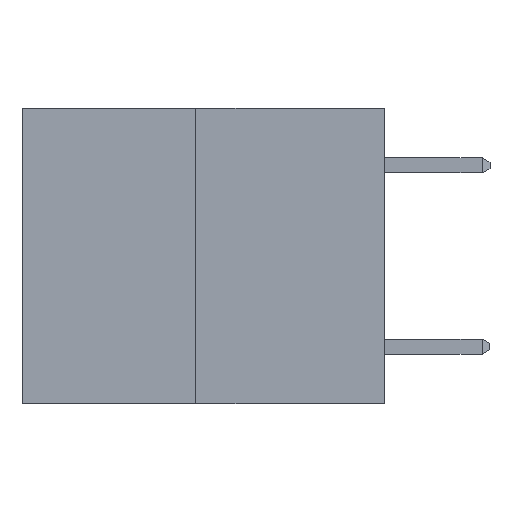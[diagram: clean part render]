
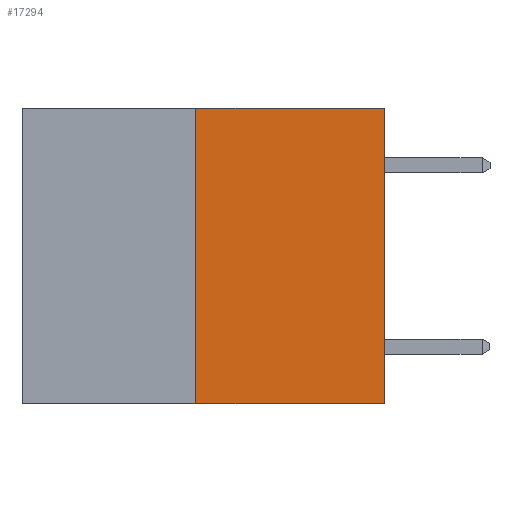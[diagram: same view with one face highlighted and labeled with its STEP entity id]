
A CAD part, left-side view. The second image highlights one B-rep face of the part: STEP entity #17294.
In plain terms, the highlighted planar face has unit normal (-1, 0, 0).
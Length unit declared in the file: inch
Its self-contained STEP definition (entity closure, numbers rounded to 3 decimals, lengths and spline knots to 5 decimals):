
#52 = ORIENTED_EDGE ( 'NONE', *, *, #888, .T. ) ;
#299 = VECTOR ( 'NONE', #5198, 39.37008 ) ;
#314 = PLANE ( 'NONE',  #11941 ) ;
#888 = EDGE_CURVE ( 'NONE', #15731, #8201, #12109, .T. ) ;
#910 = VECTOR ( 'NONE', #12872, 39.37008 ) ;
#929 = VECTOR ( 'NONE', #8258, 39.37008 ) ;
#2021 = CARTESIAN_POINT ( 'NONE',  ( 0., 0.6, -0.49 ) ) ;
#2401 = EDGE_CURVE ( 'NONE', #10324, #6937, #10796, .T. ) ;
#4137 = CARTESIAN_POINT ( 'NONE',  ( 0., 0.6, 0. ) ) ;
#4803 = CARTESIAN_POINT ( 'NONE',  ( 0., 0., 0. ) ) ;
#4825 = ORIENTED_EDGE ( 'NONE', *, *, #16258, .T. ) ;
#4911 = LINE ( 'NONE', #2021, #910 ) ;
#5198 = DIRECTION ( 'NONE',  ( 0., 0., 1. ) ) ;
#5587 = DIRECTION ( 'NONE',  ( 0., 0., 1. ) ) ;
#6163 = FACE_OUTER_BOUND ( 'NONE', #17118, .T. ) ;
#6379 = ORIENTED_EDGE ( 'NONE', *, *, #2401, .F. ) ;
#6402 = LINE ( 'NONE', #8570, #929 ) ;
#6937 = VERTEX_POINT ( 'NONE', #11582 ) ;
#8201 = VERTEX_POINT ( 'NONE', #9591 ) ;
#8258 = DIRECTION ( 'NONE',  ( 0., -1., 0. ) ) ;
#8570 = CARTESIAN_POINT ( 'NONE',  ( 0., 0.6, 0. ) ) ;
#9591 = CARTESIAN_POINT ( 'NONE',  ( 0., 0., 0. ) ) ;
#9701 = DIRECTION ( 'NONE',  ( 0., 0., -1. ) ) ;
#10324 = VERTEX_POINT ( 'NONE', #13040 ) ;
#10381 = VECTOR ( 'NONE', #5587, 39.37008 ) ;
#10796 = LINE ( 'NONE', #14986, #10381 ) ;
#11582 = CARTESIAN_POINT ( 'NONE',  ( 0., 0.312, 0. ) ) ;
#11941 = AXIS2_PLACEMENT_3D ( 'NONE', #4137, #12481, #9701 ) ;
#12109 = LINE ( 'NONE', #4803, #299 ) ;
#12481 = DIRECTION ( 'NONE',  ( 1., 0., 0. ) ) ;
#12675 = CARTESIAN_POINT ( 'NONE',  ( 0., 0., -0.49 ) ) ;
#12872 = DIRECTION ( 'NONE',  ( 0., -1., 0. ) ) ;
#13040 = CARTESIAN_POINT ( 'NONE',  ( 0., 0.312, -0.49 ) ) ;
#14986 = CARTESIAN_POINT ( 'NONE',  ( 0., 0.312, -0.49 ) ) ;
#15731 = VERTEX_POINT ( 'NONE', #12675 ) ;
#16125 = EDGE_CURVE ( 'NONE', #6937, #8201, #6402, .T. ) ;
#16258 = EDGE_CURVE ( 'NONE', #10324, #15731, #4911, .T. ) ;
#17118 = EDGE_LOOP ( 'NONE', ( #6379, #4825, #52, #17420 ) ) ;
#17294 = ADVANCED_FACE ( 'NONE', ( #6163 ), #314, .F. ) ;
#17420 = ORIENTED_EDGE ( 'NONE', *, *, #16125, .F. ) ;
